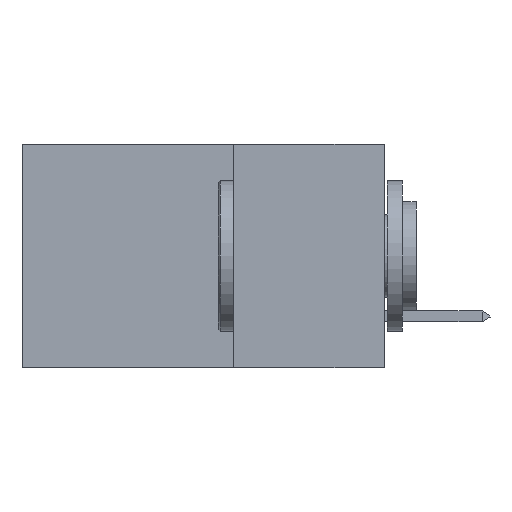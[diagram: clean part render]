
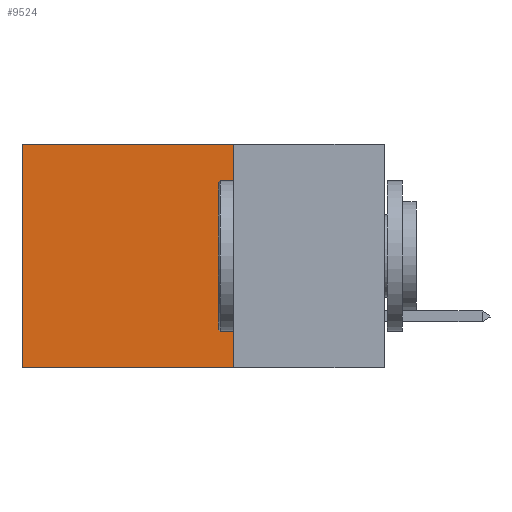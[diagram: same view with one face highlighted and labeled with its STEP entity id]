
A CAD part, left-side view. The second image highlights one B-rep face of the part: STEP entity #9524.
In plain terms, the highlighted planar face has unit normal (-1, 0, 0).
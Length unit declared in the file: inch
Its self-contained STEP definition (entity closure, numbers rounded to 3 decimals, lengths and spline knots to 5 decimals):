
#7 = FACE_OUTER_BOUND ( 'NONE', #3030, .T. ) ;
#973 = DIRECTION ( 'NONE',  ( 0., 0., -1. ) ) ;
#1192 = CARTESIAN_POINT ( 'NONE',  ( 0.2875, 0.6, -0.37 ) ) ;
#2689 = ORIENTED_EDGE ( 'NONE', *, *, #6577, .F. ) ;
#3030 = EDGE_LOOP ( 'NONE', ( #6632, #13411, #2689, #8682 ) ) ;
#4086 = VECTOR ( 'NONE', #4903, 39.37008 ) ;
#4805 = VERTEX_POINT ( 'NONE', #1192 ) ;
#4835 = CARTESIAN_POINT ( 'NONE',  ( 0.2875, 0.25, 0. ) ) ;
#4903 = DIRECTION ( 'NONE',  ( 0., 0., -1. ) ) ;
#5411 = CARTESIAN_POINT ( 'NONE',  ( 0.2875, 0.25, -0.37 ) ) ;
#5732 = EDGE_CURVE ( 'NONE', #10393, #4805, #16109, .T. ) ;
#5995 = CARTESIAN_POINT ( 'NONE',  ( 0.2875, 0.25, -0.37 ) ) ;
#6117 = DIRECTION ( 'NONE',  ( 0., 0., -1. ) ) ;
#6577 = EDGE_CURVE ( 'NONE', #9929, #15752, #10980, .T. ) ;
#6632 = ORIENTED_EDGE ( 'NONE', *, *, #5732, .T. ) ;
#6719 = CARTESIAN_POINT ( 'NONE',  ( 0.2875, 0.6, 0. ) ) ;
#7924 = LINE ( 'NONE', #5995, #8141 ) ;
#8141 = VECTOR ( 'NONE', #14800, 39.37008 ) ;
#8230 = EDGE_CURVE ( 'NONE', #15752, #4805, #7924, .T. ) ;
#8507 = DIRECTION ( 'NONE',  ( 1., 0., 0. ) ) ;
#8682 = ORIENTED_EDGE ( 'NONE', *, *, #13114, .T. ) ;
#8984 = VECTOR ( 'NONE', #6117, 39.37008 ) ;
#8988 = CARTESIAN_POINT ( 'NONE',  ( 0.2875, 0.25, 0. ) ) ;
#9524 = ADVANCED_FACE ( 'NONE', ( #7 ), #11006, .F. ) ;
#9816 = CARTESIAN_POINT ( 'NONE',  ( 0.2875, 0.6, 0. ) ) ;
#9929 = VERTEX_POINT ( 'NONE', #8988 ) ;
#10393 = VERTEX_POINT ( 'NONE', #6719 ) ;
#10479 = DIRECTION ( 'NONE',  ( 0., 1., 0. ) ) ;
#10980 = LINE ( 'NONE', #4835, #8984 ) ;
#11006 = PLANE ( 'NONE',  #12132 ) ;
#11239 = VECTOR ( 'NONE', #10479, 39.37008 ) ;
#12132 = AXIS2_PLACEMENT_3D ( 'NONE', #16048, #8507, #973 ) ;
#13114 = EDGE_CURVE ( 'NONE', #9929, #10393, #14552, .T. ) ;
#13411 = ORIENTED_EDGE ( 'NONE', *, *, #8230, .F. ) ;
#14197 = CARTESIAN_POINT ( 'NONE',  ( 0.2875, 0.25, 0. ) ) ;
#14552 = LINE ( 'NONE', #14197, #11239 ) ;
#14800 = DIRECTION ( 'NONE',  ( 0., 1., 0. ) ) ;
#15752 = VERTEX_POINT ( 'NONE', #5411 ) ;
#16048 = CARTESIAN_POINT ( 'NONE',  ( 0.2875, 0.25, 0. ) ) ;
#16109 = LINE ( 'NONE', #9816, #4086 ) ;
